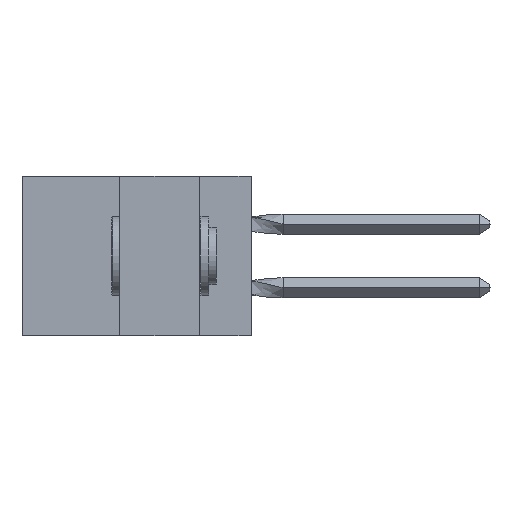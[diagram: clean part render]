
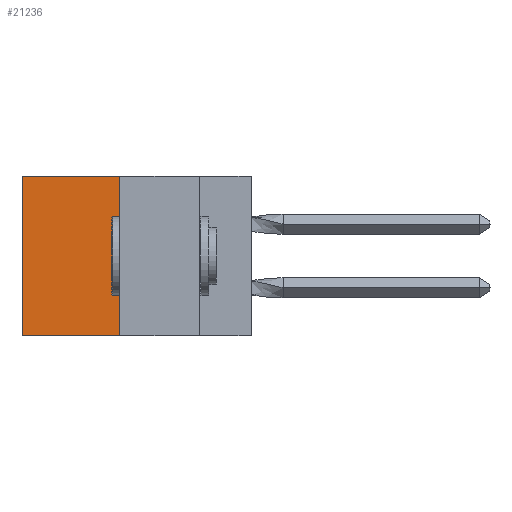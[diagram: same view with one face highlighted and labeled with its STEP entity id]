
A CAD part, left-side view. The second image highlights one B-rep face of the part: STEP entity #21236.
In plain terms, the highlighted planar face has unit normal (-1, 0, 0).
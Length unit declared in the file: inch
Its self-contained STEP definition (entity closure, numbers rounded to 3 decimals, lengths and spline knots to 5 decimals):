
#1108 = CARTESIAN_POINT ( 'NONE',  ( 0.305, 0.413, -0.5 ) ) ;
#1190 = DIRECTION ( 'NONE',  ( 0., 0., -1. ) ) ;
#2296 = ORIENTED_EDGE ( 'NONE', *, *, #13971, .T. ) ;
#3232 = VERTEX_POINT ( 'NONE', #5343 ) ;
#3422 = PLANE ( 'NONE',  #11793 ) ;
#4070 = VECTOR ( 'NONE', #9857, 39.37008 ) ;
#5095 = CARTESIAN_POINT ( 'NONE',  ( 0.305, 0.413, -0.5 ) ) ;
#5343 = CARTESIAN_POINT ( 'NONE',  ( 0.305, 0.413, 0. ) ) ;
#5422 = FACE_OUTER_BOUND ( 'NONE', #8139, .T. ) ;
#6338 = ORIENTED_EDGE ( 'NONE', *, *, #7261, .T. ) ;
#6440 = VERTEX_POINT ( 'NONE', #9602 ) ;
#6650 = DIRECTION ( 'NONE',  ( 0., 1., 0. ) ) ;
#6892 = VECTOR ( 'NONE', #17496, 39.37008 ) ;
#7261 = EDGE_CURVE ( 'NONE', #3232, #6440, #10743, .T. ) ;
#8139 = EDGE_LOOP ( 'NONE', ( #2296, #19746, #17296, #6338 ) ) ;
#9602 = CARTESIAN_POINT ( 'NONE',  ( 0.305, 0.72, 0. ) ) ;
#9857 = DIRECTION ( 'NONE',  ( 0., 0., -1. ) ) ;
#10743 = LINE ( 'NONE', #24869, #19370 ) ;
#11575 = DIRECTION ( 'NONE',  ( 1., 0., 0. ) ) ;
#11793 = AXIS2_PLACEMENT_3D ( 'NONE', #13464, #11575, #1190 ) ;
#13464 = CARTESIAN_POINT ( 'NONE',  ( 0.305, 0.413, -0.5 ) ) ;
#13971 = EDGE_CURVE ( 'NONE', #6440, #15414, #15230, .T. ) ;
#14019 = CARTESIAN_POINT ( 'NONE',  ( 0.305, 0.72, -0.5 ) ) ;
#15230 = LINE ( 'NONE', #14019, #4070 ) ;
#15414 = VERTEX_POINT ( 'NONE', #21530 ) ;
#16003 = VECTOR ( 'NONE', #23546, 39.37008 ) ;
#17296 = ORIENTED_EDGE ( 'NONE', *, *, #18850, .F. ) ;
#17381 = VERTEX_POINT ( 'NONE', #1108 ) ;
#17496 = DIRECTION ( 'NONE',  ( 0., 1., 0. ) ) ;
#18850 = EDGE_CURVE ( 'NONE', #3232, #17381, #19871, .T. ) ;
#19370 = VECTOR ( 'NONE', #6650, 39.37008 ) ;
#19527 = CARTESIAN_POINT ( 'NONE',  ( 0.305, 0.413, -0.5 ) ) ;
#19680 = LINE ( 'NONE', #5095, #6892 ) ;
#19746 = ORIENTED_EDGE ( 'NONE', *, *, #24791, .F. ) ;
#19871 = LINE ( 'NONE', #19527, #16003 ) ;
#21236 = ADVANCED_FACE ( 'NONE', ( #5422 ), #3422, .F. ) ;
#21530 = CARTESIAN_POINT ( 'NONE',  ( 0.305, 0.72, -0.5 ) ) ;
#23546 = DIRECTION ( 'NONE',  ( 0., 0., -1. ) ) ;
#24791 = EDGE_CURVE ( 'NONE', #17381, #15414, #19680, .T. ) ;
#24869 = CARTESIAN_POINT ( 'NONE',  ( 0.305, 0.413, 0. ) ) ;
